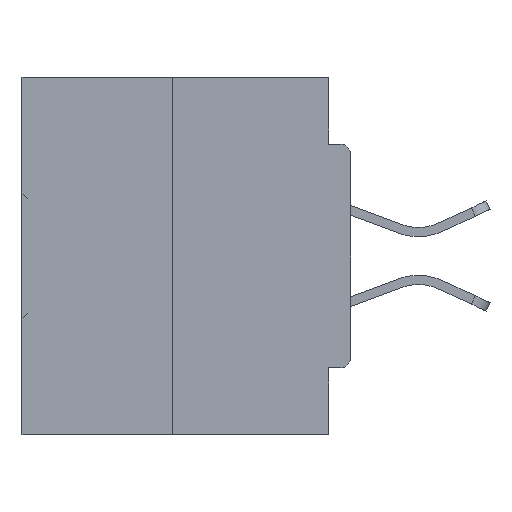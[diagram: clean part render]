
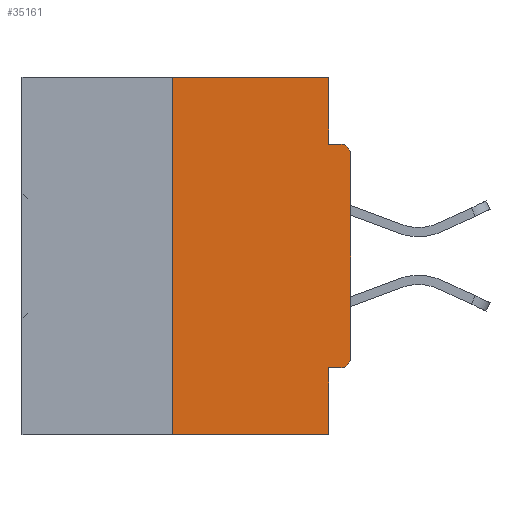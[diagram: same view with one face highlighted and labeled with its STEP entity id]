
A CAD part, left-side view. The second image highlights one B-rep face of the part: STEP entity #35161.
In plain terms, the highlighted planar face has unit normal (-1, 0, 0).
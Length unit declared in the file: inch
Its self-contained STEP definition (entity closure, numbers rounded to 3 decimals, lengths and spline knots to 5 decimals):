
#558 = EDGE_CURVE ( 'NONE', #12221, #41471, #18197, .T. ) ;
#701 = EDGE_CURVE ( 'NONE', #3617, #30866, #43238, .T. ) ;
#798 = CARTESIAN_POINT ( 'NONE',  ( 0., 0., -0.4065 ) ) ;
#1288 = DIRECTION ( 'NONE',  ( 0., 1., 0. ) ) ;
#2589 = CARTESIAN_POINT ( 'NONE',  ( 0., 0.46, 0. ) ) ;
#3184 = VECTOR ( 'NONE', #24545, 39.37008 ) ;
#3617 = VERTEX_POINT ( 'NONE', #14174 ) ;
#3799 = EDGE_CURVE ( 'NONE', #21319, #3617, #23846, .T. ) ;
#5137 = VECTOR ( 'NONE', #1288, 39.37008 ) ;
#5393 = EDGE_CURVE ( 'NONE', #29690, #12684, #15880, .T. ) ;
#6997 = ORIENTED_EDGE ( 'NONE', *, *, #5393, .F. ) ;
#7795 = VERTEX_POINT ( 'NONE', #15363 ) ;
#8523 = ORIENTED_EDGE ( 'NONE', *, *, #35139, .F. ) ;
#8681 = AXIS2_PLACEMENT_3D ( 'NONE', #29833, #40952, #40809 ) ;
#9808 = ORIENTED_EDGE ( 'NONE', *, *, #701, .F. ) ;
#11525 = DIRECTION ( 'NONE',  ( 0., -1., 0. ) ) ;
#11534 = LINE ( 'NONE', #22923, #20054 ) ;
#12042 = ORIENTED_EDGE ( 'NONE', *, *, #38855, .T. ) ;
#12221 = VERTEX_POINT ( 'NONE', #27988 ) ;
#12684 = VERTEX_POINT ( 'NONE', #21494 ) ;
#13037 = ORIENTED_EDGE ( 'NONE', *, *, #3799, .F. ) ;
#13642 = CARTESIAN_POINT ( 'NONE',  ( 0., 0.031, -0.5 ) ) ;
#14174 = CARTESIAN_POINT ( 'NONE',  ( 0., 0.031, -0.0935 ) ) ;
#14653 = CARTESIAN_POINT ( 'NONE',  ( 0., 0.25, 0. ) ) ;
#15217 = VECTOR ( 'NONE', #31763, 39.37008 ) ;
#15363 = CARTESIAN_POINT ( 'NONE',  ( 0., 0.031, -0.5 ) ) ;
#15668 = DIRECTION ( 'NONE',  ( 0., 0., -1. ) ) ;
#15759 = DIRECTION ( 'NONE',  ( 0., 0., 1. ) ) ;
#15880 = LINE ( 'NONE', #798, #5137 ) ;
#17127 = CARTESIAN_POINT ( 'NONE',  ( 0., 0., -0.3915 ) ) ;
#18197 = LINE ( 'NONE', #14653, #35806 ) ;
#20054 = VECTOR ( 'NONE', #15759, 39.37008 ) ;
#20335 = EDGE_CURVE ( 'NONE', #12221, #7795, #44247, .T. ) ;
#20673 = DIRECTION ( 'NONE',  ( 1., 0., 0. ) ) ;
#20825 = CARTESIAN_POINT ( 'NONE',  ( 0., 0.031, 0. ) ) ;
#21319 = VERTEX_POINT ( 'NONE', #20825 ) ;
#21494 = CARTESIAN_POINT ( 'NONE',  ( 0., 0.031, -0.4065 ) ) ;
#21713 = EDGE_CURVE ( 'NONE', #34616, #30866, #25925, .T. ) ;
#22923 = CARTESIAN_POINT ( 'NONE',  ( 0., 0., 0. ) ) ;
#23611 = EDGE_CURVE ( 'NONE', #41471, #21319, #41841, .T. ) ;
#23846 = LINE ( 'NONE', #26732, #25579 ) ;
#23996 = PLANE ( 'NONE',  #32218 ) ;
#24545 = DIRECTION ( 'NONE',  ( 0., -1., 0. ) ) ;
#25080 = CARTESIAN_POINT ( 'NONE',  ( 0., 0.46, -0.5 ) ) ;
#25177 = LINE ( 'NONE', #13642, #33696 ) ;
#25579 = VECTOR ( 'NONE', #27051, 39.37008 ) ;
#25767 = EDGE_LOOP ( 'NONE', ( #42548, #26111, #43668, #8523, #6997, #44616, #12042, #44995, #9808, #13037 ) ) ;
#25925 = CIRCLE ( 'NONE', #40125, 0.015 ) ;
#26111 = ORIENTED_EDGE ( 'NONE', *, *, #558, .F. ) ;
#26732 = CARTESIAN_POINT ( 'NONE',  ( 0., 0.031, 0. ) ) ;
#26809 = CARTESIAN_POINT ( 'NONE',  ( 0., 0.015, -0.1085 ) ) ;
#27051 = DIRECTION ( 'NONE',  ( 0., 0., -1. ) ) ;
#27988 = CARTESIAN_POINT ( 'NONE',  ( 0., 0.25, -0.5 ) ) ;
#28905 = CIRCLE ( 'NONE', #8681, 0.015 ) ;
#29690 = VERTEX_POINT ( 'NONE', #30563 ) ;
#29833 = CARTESIAN_POINT ( 'NONE',  ( 0., 0.015, -0.3915 ) ) ;
#30288 = FACE_OUTER_BOUND ( 'NONE', #25767, .T. ) ;
#30563 = CARTESIAN_POINT ( 'NONE',  ( 0., 0.015, -0.4065 ) ) ;
#30734 = VECTOR ( 'NONE', #11525, 39.37008 ) ;
#30866 = VERTEX_POINT ( 'NONE', #45402 ) ;
#31463 = DIRECTION ( 'NONE',  ( 0., 0., -1. ) ) ;
#31763 = DIRECTION ( 'NONE',  ( 0., -1., 0. ) ) ;
#32218 = AXIS2_PLACEMENT_3D ( 'NONE', #2589, #20673, #42303 ) ;
#33696 = VECTOR ( 'NONE', #31463, 39.37008 ) ;
#34616 = VERTEX_POINT ( 'NONE', #42823 ) ;
#35139 = EDGE_CURVE ( 'NONE', #12684, #7795, #25177, .T. ) ;
#35161 = ADVANCED_FACE ( 'NONE', ( #30288 ), #23996, .F. ) ;
#35806 = VECTOR ( 'NONE', #43016, 39.37008 ) ;
#35953 = CARTESIAN_POINT ( 'NONE',  ( 0., 0.46, 0. ) ) ;
#38855 = EDGE_CURVE ( 'NONE', #44184, #34616, #11534, .T. ) ;
#40125 = AXIS2_PLACEMENT_3D ( 'NONE', #26809, #45263, #15668 ) ;
#40809 = DIRECTION ( 'NONE',  ( 0., 0., -1. ) ) ;
#40952 = DIRECTION ( 'NONE',  ( -1., 0., 0. ) ) ;
#41471 = VERTEX_POINT ( 'NONE', #42036 ) ;
#41761 = EDGE_CURVE ( 'NONE', #29690, #44184, #28905, .T. ) ;
#41841 = LINE ( 'NONE', #35953, #3184 ) ;
#42036 = CARTESIAN_POINT ( 'NONE',  ( 0., 0.25, 0. ) ) ;
#42303 = DIRECTION ( 'NONE',  ( 0., 0., -1. ) ) ;
#42548 = ORIENTED_EDGE ( 'NONE', *, *, #23611, .F. ) ;
#42823 = CARTESIAN_POINT ( 'NONE',  ( 0., 0., -0.1085 ) ) ;
#43016 = DIRECTION ( 'NONE',  ( 0., 0., 1. ) ) ;
#43238 = LINE ( 'NONE', #43950, #30734 ) ;
#43668 = ORIENTED_EDGE ( 'NONE', *, *, #20335, .T. ) ;
#43950 = CARTESIAN_POINT ( 'NONE',  ( 0., 0., -0.0935 ) ) ;
#44184 = VERTEX_POINT ( 'NONE', #17127 ) ;
#44247 = LINE ( 'NONE', #25080, #15217 ) ;
#44616 = ORIENTED_EDGE ( 'NONE', *, *, #41761, .T. ) ;
#44995 = ORIENTED_EDGE ( 'NONE', *, *, #21713, .T. ) ;
#45263 = DIRECTION ( 'NONE',  ( -1., 0., 0. ) ) ;
#45402 = CARTESIAN_POINT ( 'NONE',  ( 0., 0.015, -0.0935 ) ) ;
